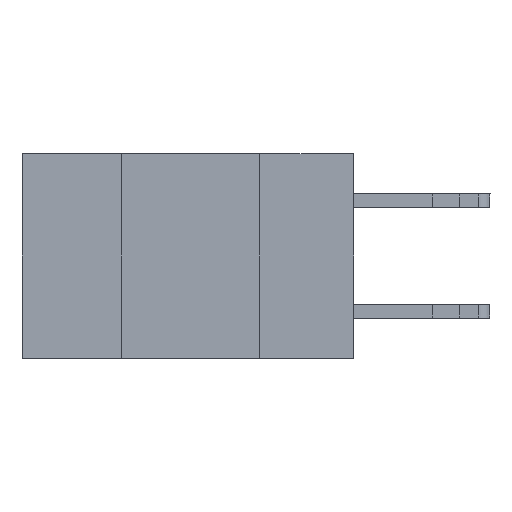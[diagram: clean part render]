
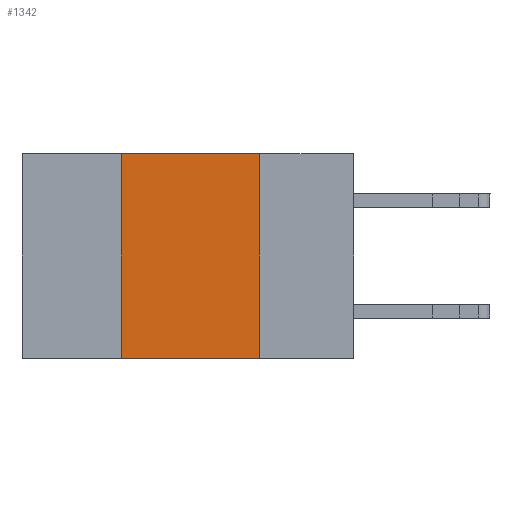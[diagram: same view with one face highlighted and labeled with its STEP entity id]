
A CAD part, left-side view. The second image highlights one B-rep face of the part: STEP entity #1342.
In plain terms, the highlighted planar face has unit normal (-1, 0, 0).
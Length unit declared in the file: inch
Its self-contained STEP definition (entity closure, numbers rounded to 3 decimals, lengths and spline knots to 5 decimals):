
#25 = EDGE_LOOP ( 'NONE', ( #468, #24645, #658, #11479 ) ) ;
#468 = ORIENTED_EDGE ( 'NONE', *, *, #19662, .F. ) ;
#480 = DIRECTION ( 'NONE',  ( 0., 0., -1. ) ) ;
#658 = ORIENTED_EDGE ( 'NONE', *, *, #21196, .F. ) ;
#1342 = ADVANCED_FACE ( 'NONE', ( #21612 ), #23377, .F. ) ;
#1960 = CARTESIAN_POINT ( 'NONE',  ( 0., 0.42, -0.37 ) ) ;
#2040 = CARTESIAN_POINT ( 'NONE',  ( 0., 0.6, 0. ) ) ;
#2752 = VECTOR ( 'NONE', #3312, 39.37008 ) ;
#3312 = DIRECTION ( 'NONE',  ( 0., 0., 1. ) ) ;
#3344 = VERTEX_POINT ( 'NONE', #23596 ) ;
#4213 = AXIS2_PLACEMENT_3D ( 'NONE', #6075, #13796, #480 ) ;
#5293 = EDGE_CURVE ( 'NONE', #14006, #18270, #9035, .T. ) ;
#6075 = CARTESIAN_POINT ( 'NONE',  ( 0., 0.6, 0. ) ) ;
#8932 = EDGE_CURVE ( 'NONE', #15055, #3344, #21260, .T. ) ;
#9035 = LINE ( 'NONE', #14334, #24376 ) ;
#11479 = ORIENTED_EDGE ( 'NONE', *, *, #5293, .T. ) ;
#12944 = CARTESIAN_POINT ( 'NONE',  ( 0., 0.42, 0. ) ) ;
#13796 = DIRECTION ( 'NONE',  ( 1., 0., 0. ) ) ;
#14006 = VERTEX_POINT ( 'NONE', #1960 ) ;
#14334 = CARTESIAN_POINT ( 'NONE',  ( 0., 0.6, -0.37 ) ) ;
#14440 = LINE ( 'NONE', #20133, #15193 ) ;
#15055 = VERTEX_POINT ( 'NONE', #22475 ) ;
#15193 = VECTOR ( 'NONE', #22143, 39.37008 ) ;
#15738 = VECTOR ( 'NONE', #23165, 39.37008 ) ;
#18270 = VERTEX_POINT ( 'NONE', #19449 ) ;
#19449 = CARTESIAN_POINT ( 'NONE',  ( 0., 0.17, -0.37 ) ) ;
#19662 = EDGE_CURVE ( 'NONE', #3344, #18270, #14440, .T. ) ;
#20133 = CARTESIAN_POINT ( 'NONE',  ( 0., 0.17, 0. ) ) ;
#21196 = EDGE_CURVE ( 'NONE', #14006, #15055, #22522, .T. ) ;
#21260 = LINE ( 'NONE', #2040, #15738 ) ;
#21612 = FACE_OUTER_BOUND ( 'NONE', #25, .T. ) ;
#22025 = DIRECTION ( 'NONE',  ( 0., -1., 0. ) ) ;
#22143 = DIRECTION ( 'NONE',  ( 0., 0., -1. ) ) ;
#22475 = CARTESIAN_POINT ( 'NONE',  ( 0., 0.42, 0. ) ) ;
#22522 = LINE ( 'NONE', #12944, #2752 ) ;
#23165 = DIRECTION ( 'NONE',  ( 0., -1., 0. ) ) ;
#23377 = PLANE ( 'NONE',  #4213 ) ;
#23596 = CARTESIAN_POINT ( 'NONE',  ( 0., 0.17, 0. ) ) ;
#24376 = VECTOR ( 'NONE', #22025, 39.37008 ) ;
#24645 = ORIENTED_EDGE ( 'NONE', *, *, #8932, .F. ) ;
